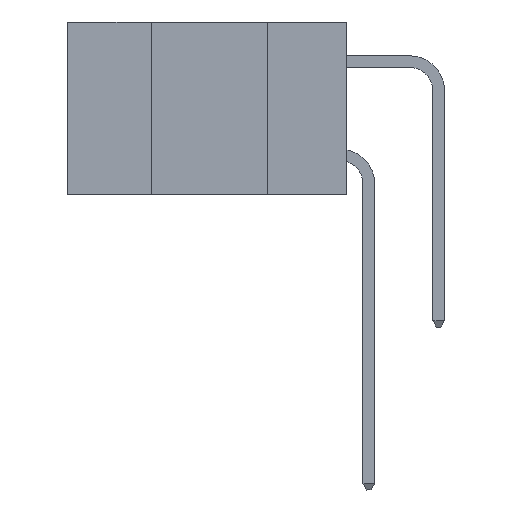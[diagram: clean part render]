
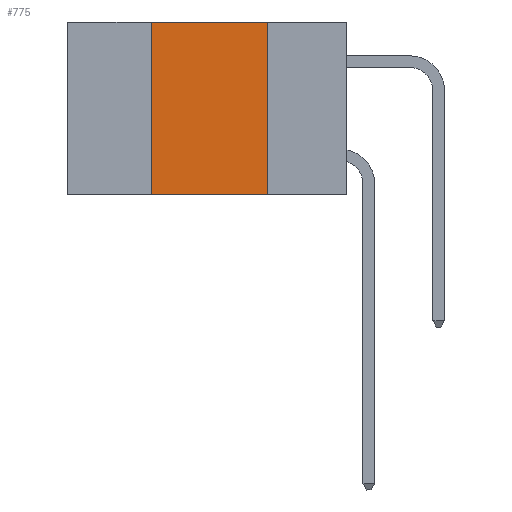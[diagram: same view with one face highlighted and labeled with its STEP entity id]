
A CAD part, left-side view. The second image highlights one B-rep face of the part: STEP entity #775.
In plain terms, the highlighted planar face has unit normal (-1, 0, 0).
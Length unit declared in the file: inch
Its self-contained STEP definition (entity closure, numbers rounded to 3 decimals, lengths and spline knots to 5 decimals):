
#775 = ADVANCED_FACE ( 'NONE', ( #5980 ), #25281, .F. ) ;
#1895 = CARTESIAN_POINT ( 'NONE',  ( 0., 0.17, 0. ) ) ;
#2073 = VERTEX_POINT ( 'NONE', #17434 ) ;
#2813 = DIRECTION ( 'NONE',  ( 0., -1., 0. ) ) ;
#3620 = CARTESIAN_POINT ( 'NONE',  ( 0., 0.42, 0. ) ) ;
#3797 = DIRECTION ( 'NONE',  ( 0., 0., -1. ) ) ;
#3978 = ORIENTED_EDGE ( 'NONE', *, *, #26668, .F. ) ;
#4848 = ORIENTED_EDGE ( 'NONE', *, *, #4964, .F. ) ;
#4915 = LINE ( 'NONE', #9077, #17905 ) ;
#4964 = EDGE_CURVE ( 'NONE', #14849, #6715, #6604, .T. ) ;
#5758 = ORIENTED_EDGE ( 'NONE', *, *, #21082, .T. ) ;
#5980 = FACE_OUTER_BOUND ( 'NONE', #12890, .T. ) ;
#6604 = LINE ( 'NONE', #3620, #13397 ) ;
#6715 = VERTEX_POINT ( 'NONE', #17705 ) ;
#7832 = ORIENTED_EDGE ( 'NONE', *, *, #20457, .F. ) ;
#9077 = CARTESIAN_POINT ( 'NONE',  ( 0., 0.6, -0.37 ) ) ;
#9391 = DIRECTION ( 'NONE',  ( 0., -1., 0. ) ) ;
#10086 = VERTEX_POINT ( 'NONE', #16350 ) ;
#10109 = LINE ( 'NONE', #1895, #16262 ) ;
#12532 = CARTESIAN_POINT ( 'NONE',  ( 0., 0.42, -0.37 ) ) ;
#12890 = EDGE_LOOP ( 'NONE', ( #3978, #7832, #4848, #5758 ) ) ;
#13397 = VECTOR ( 'NONE', #20308, 39.37008 ) ;
#14839 = CARTESIAN_POINT ( 'NONE',  ( 0., 0.6, 0. ) ) ;
#14849 = VERTEX_POINT ( 'NONE', #12532 ) ;
#15976 = VECTOR ( 'NONE', #9391, 39.37008 ) ;
#16262 = VECTOR ( 'NONE', #3797, 39.37008 ) ;
#16350 = CARTESIAN_POINT ( 'NONE',  ( 0., 0.17, 0. ) ) ;
#17434 = CARTESIAN_POINT ( 'NONE',  ( 0., 0.17, -0.37 ) ) ;
#17705 = CARTESIAN_POINT ( 'NONE',  ( 0., 0.42, 0. ) ) ;
#17794 = AXIS2_PLACEMENT_3D ( 'NONE', #14839, #19288, #19016 ) ;
#17905 = VECTOR ( 'NONE', #2813, 39.37008 ) ;
#19016 = DIRECTION ( 'NONE',  ( 0., 0., -1. ) ) ;
#19288 = DIRECTION ( 'NONE',  ( 1., 0., 0. ) ) ;
#20308 = DIRECTION ( 'NONE',  ( 0., 0., 1. ) ) ;
#20457 = EDGE_CURVE ( 'NONE', #6715, #10086, #21494, .T. ) ;
#21082 = EDGE_CURVE ( 'NONE', #14849, #2073, #4915, .T. ) ;
#21494 = LINE ( 'NONE', #25624, #15976 ) ;
#25281 = PLANE ( 'NONE',  #17794 ) ;
#25624 = CARTESIAN_POINT ( 'NONE',  ( 0., 0.6, 0. ) ) ;
#26668 = EDGE_CURVE ( 'NONE', #10086, #2073, #10109, .T. ) ;
